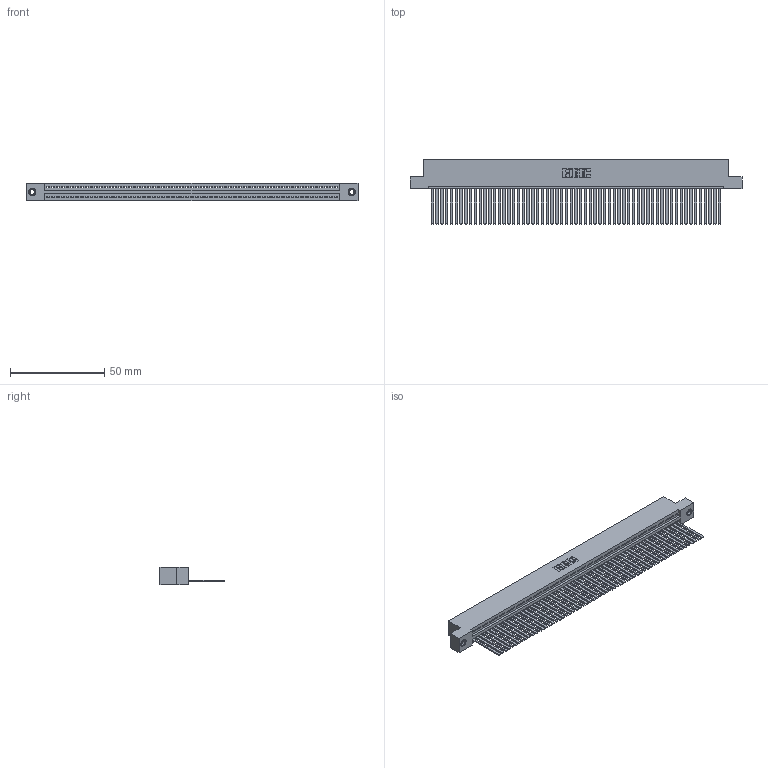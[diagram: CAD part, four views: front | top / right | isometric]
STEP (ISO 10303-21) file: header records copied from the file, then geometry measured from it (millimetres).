
FILE_DESCRIPTION (( 'STEP AP203' ), '1' );
FILE_NAME ('395-061-544-107.STEP', '2019-10-24T15:59:19', ( '' ), ( '' ), 'SwSTEP 2.0', 'SolidWorks 2016', '' );
FILE_SCHEMA (( 'CONFIG_CONTROL_DESIGN' ));
Length unit declared in the file: inch
Products named in the file (4): 395-061-544-107; 345 Part_Flush Mounting Lugs - 0.156 Dia-TI; 345-292-001_345-293-144; 345-250-001_345-250-005-103
Assembly tree (64 placements, depth 2):
  395-061-544-107
    345 Part_Flush Mounting Lugs - 0.156 Dia-TI
    345-292-001_345-293-144  x61
    345-250-001_345-250-005-103  x2
Bounding box: 176.15 x 33.96 x 9.4 mm (x, y, z)
Volume: 17579.4 mm3; surface area: 25773.1 mm2
Topology: 64 solids, 64 shells, 3358 faces, 10115 edges, 6654 vertices
Faces by surface type: plane 2308, cylinder 1034, cone 12, torus 4
Entity records: 44354 total; most frequent: CARTESIAN_POINT 7662, ORIENTED_EDGE 7650, DIRECTION 6689, EDGE_CURVE 3825, LINE 3433, VECTOR 3433, VERTEX_POINT 2544, AXIS2_PLACEMENT_3D 1628
